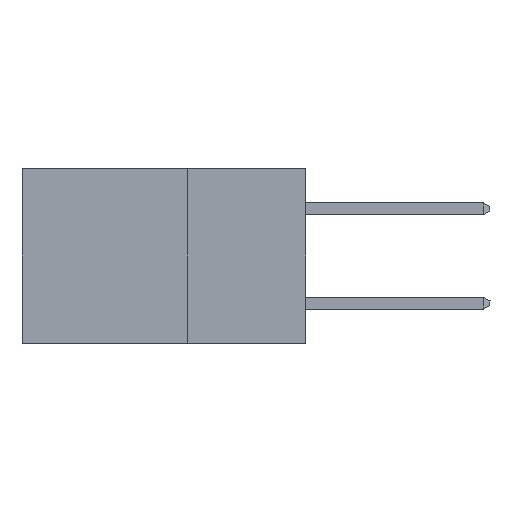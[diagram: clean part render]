
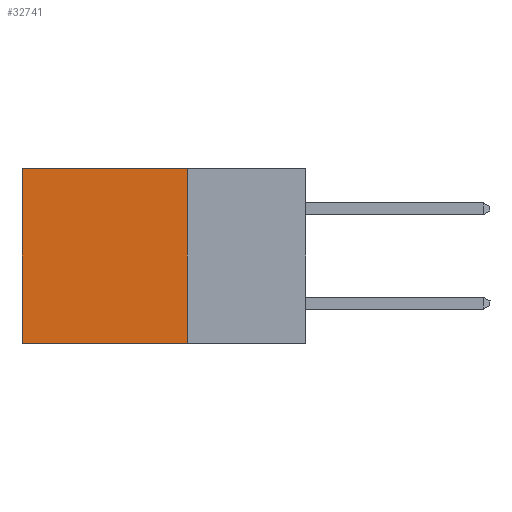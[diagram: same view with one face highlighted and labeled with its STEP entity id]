
A CAD part, left-side view. The second image highlights one B-rep face of the part: STEP entity #32741.
In plain terms, the highlighted planar face has unit normal (-1, 0, 0).
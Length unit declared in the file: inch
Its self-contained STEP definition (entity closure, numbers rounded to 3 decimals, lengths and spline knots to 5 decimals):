
#1039 = ORIENTED_EDGE ( 'NONE', *, *, #17451, .F. ) ;
#1506 = CARTESIAN_POINT ( 'NONE',  ( 0.298, 0.25, 0. ) ) ;
#1795 = VECTOR ( 'NONE', #23576, 39.37008 ) ;
#3037 = LINE ( 'NONE', #20918, #1795 ) ;
#3894 = ORIENTED_EDGE ( 'NONE', *, *, #33774, .T. ) ;
#5260 = CARTESIAN_POINT ( 'NONE',  ( 0.298, 0.25, -0.37 ) ) ;
#5696 = AXIS2_PLACEMENT_3D ( 'NONE', #24182, #6075, #16562 ) ;
#6075 = DIRECTION ( 'NONE',  ( 1., 0., 0. ) ) ;
#10540 = EDGE_LOOP ( 'NONE', ( #19053, #11594, #1039, #3894 ) ) ;
#11479 = VECTOR ( 'NONE', #16277, 39.37008 ) ;
#11594 = ORIENTED_EDGE ( 'NONE', *, *, #27228, .F. ) ;
#11754 = DIRECTION ( 'NONE',  ( 0., 1., 0. ) ) ;
#12653 = VECTOR ( 'NONE', #11754, 39.37008 ) ;
#12887 = DIRECTION ( 'NONE',  ( 0., 0., -1. ) ) ;
#13716 = CARTESIAN_POINT ( 'NONE',  ( 0.298, 0.25, 0. ) ) ;
#13758 = PLANE ( 'NONE',  #5696 ) ;
#14176 = CARTESIAN_POINT ( 'NONE',  ( 0.298, 0.25, -0.37 ) ) ;
#14356 = LINE ( 'NONE', #13716, #11479 ) ;
#16277 = DIRECTION ( 'NONE',  ( 0., 0., -1. ) ) ;
#16490 = VERTEX_POINT ( 'NONE', #23750 ) ;
#16562 = DIRECTION ( 'NONE',  ( 0., 0., -1. ) ) ;
#17031 = EDGE_CURVE ( 'NONE', #32878, #16490, #27693, .T. ) ;
#17360 = CARTESIAN_POINT ( 'NONE',  ( 0.298, 0.6, 0. ) ) ;
#17451 = EDGE_CURVE ( 'NONE', #28459, #19297, #14356, .T. ) ;
#18884 = FACE_OUTER_BOUND ( 'NONE', #10540, .T. ) ;
#19053 = ORIENTED_EDGE ( 'NONE', *, *, #17031, .T. ) ;
#19297 = VERTEX_POINT ( 'NONE', #5260 ) ;
#19830 = VECTOR ( 'NONE', #12887, 39.37008 ) ;
#20918 = CARTESIAN_POINT ( 'NONE',  ( 0.298, 0.25, 0. ) ) ;
#23576 = DIRECTION ( 'NONE',  ( 0., 1., 0. ) ) ;
#23750 = CARTESIAN_POINT ( 'NONE',  ( 0.298, 0.6, -0.37 ) ) ;
#24182 = CARTESIAN_POINT ( 'NONE',  ( 0.298, 0.25, 0. ) ) ;
#27228 = EDGE_CURVE ( 'NONE', #19297, #16490, #32195, .T. ) ;
#27693 = LINE ( 'NONE', #31601, #19830 ) ;
#28459 = VERTEX_POINT ( 'NONE', #1506 ) ;
#31601 = CARTESIAN_POINT ( 'NONE',  ( 0.298, 0.6, 0. ) ) ;
#32195 = LINE ( 'NONE', #14176, #12653 ) ;
#32741 = ADVANCED_FACE ( 'NONE', ( #18884 ), #13758, .F. ) ;
#32878 = VERTEX_POINT ( 'NONE', #17360 ) ;
#33774 = EDGE_CURVE ( 'NONE', #28459, #32878, #3037, .T. ) ;
